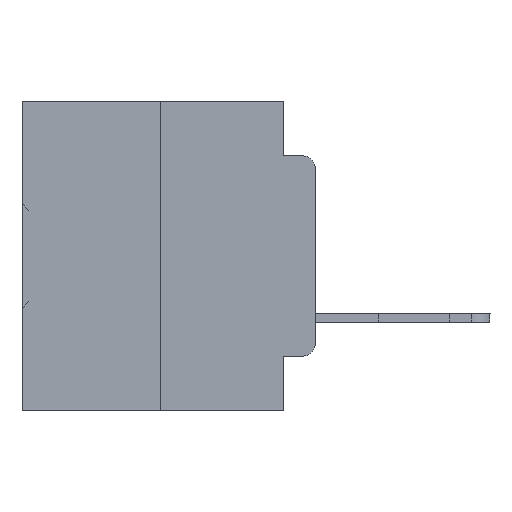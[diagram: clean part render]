
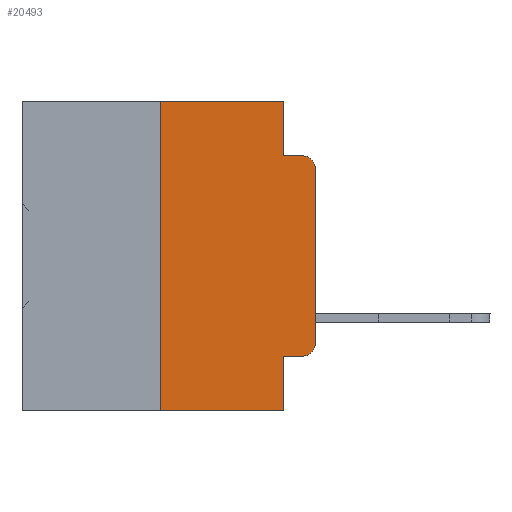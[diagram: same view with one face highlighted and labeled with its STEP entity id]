
A CAD part, left-side view. The second image highlights one B-rep face of the part: STEP entity #20493.
In plain terms, the highlighted planar face has unit normal (-1, 0, 0).
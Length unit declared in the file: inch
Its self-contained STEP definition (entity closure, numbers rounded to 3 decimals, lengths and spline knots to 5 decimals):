
#1062 = EDGE_CURVE ( 'NONE', #1080, #31317, #7346, .T. ) ;
#1080 = VERTEX_POINT ( 'NONE', #16188 ) ;
#1418 = VERTEX_POINT ( 'NONE', #6391 ) ;
#1622 = ORIENTED_EDGE ( 'NONE', *, *, #22302, .F. ) ;
#2137 = LINE ( 'NONE', #31240, #18151 ) ;
#2166 = CARTESIAN_POINT ( 'NONE',  ( 0., 0.02, -0.1085 ) ) ;
#2655 = ORIENTED_EDGE ( 'NONE', *, *, #32962, .F. ) ;
#3033 = DIRECTION ( 'NONE',  ( 0., -1., 0. ) ) ;
#3649 = ORIENTED_EDGE ( 'NONE', *, *, #21889, .F. ) ;
#4477 = DIRECTION ( 'NONE',  ( 0., 0., 1. ) ) ;
#5012 = DIRECTION ( 'NONE',  ( 0., 0., 1. ) ) ;
#5609 = DIRECTION ( 'NONE',  ( 0., 0., -1. ) ) ;
#5659 = DIRECTION ( 'NONE',  ( -1., 0., 0. ) ) ;
#5760 = EDGE_CURVE ( 'NONE', #37710, #1080, #20827, .T. ) ;
#5964 = DIRECTION ( 'NONE',  ( 0., 0., -1. ) ) ;
#6171 = LINE ( 'NONE', #17882, #10372 ) ;
#6391 = CARTESIAN_POINT ( 'NONE',  ( 0., 0.051, -0.4115 ) ) ;
#7346 = LINE ( 'NONE', #19021, #15452 ) ;
#7853 = VERTEX_POINT ( 'NONE', #30922 ) ;
#8041 = LINE ( 'NONE', #31603, #34232 ) ;
#8723 = DIRECTION ( 'NONE',  ( 0., 0., -1. ) ) ;
#8746 = AXIS2_PLACEMENT_3D ( 'NONE', #30864, #31432, #28547 ) ;
#8863 = LINE ( 'NONE', #20525, #22206 ) ;
#9950 = LINE ( 'NONE', #18746, #20154 ) ;
#10372 = VECTOR ( 'NONE', #23235, 39.37008 ) ;
#10520 = CIRCLE ( 'NONE', #31913, 0.02 ) ;
#10738 = LINE ( 'NONE', #37153, #15723 ) ;
#12020 = ORIENTED_EDGE ( 'NONE', *, *, #20349, .F. ) ;
#12160 = VERTEX_POINT ( 'NONE', #22994 ) ;
#13338 = CARTESIAN_POINT ( 'NONE',  ( 0., 0.051, 0. ) ) ;
#13588 = LINE ( 'NONE', #31182, #22371 ) ;
#15452 = VECTOR ( 'NONE', #4477, 39.37008 ) ;
#15601 = VERTEX_POINT ( 'NONE', #15735 ) ;
#15723 = VECTOR ( 'NONE', #3033, 39.37008 ) ;
#15735 = CARTESIAN_POINT ( 'NONE',  ( 0., 0.051, -0.0885 ) ) ;
#15758 = ORIENTED_EDGE ( 'NONE', *, *, #5760, .T. ) ;
#16188 = CARTESIAN_POINT ( 'NONE',  ( 0., 0., -0.3915 ) ) ;
#16746 = VERTEX_POINT ( 'NONE', #35636 ) ;
#16987 = EDGE_CURVE ( 'NONE', #30671, #15601, #8041, .T. ) ;
#17213 = EDGE_CURVE ( 'NONE', #16746, #18371, #9950, .T. ) ;
#17882 = CARTESIAN_POINT ( 'NONE',  ( 0., 0.051, -0.4115 ) ) ;
#18151 = VECTOR ( 'NONE', #5012, 39.37008 ) ;
#18371 = VERTEX_POINT ( 'NONE', #33491 ) ;
#18746 = CARTESIAN_POINT ( 'NONE',  ( 0., 0.473, -0.5 ) ) ;
#19021 = CARTESIAN_POINT ( 'NONE',  ( 0., 0., 0. ) ) ;
#20154 = VECTOR ( 'NONE', #27558, 39.37008 ) ;
#20349 = EDGE_CURVE ( 'NONE', #1418, #18371, #8863, .T. ) ;
#20493 = ADVANCED_FACE ( 'NONE', ( #24374 ), #22432, .F. ) ;
#20525 = CARTESIAN_POINT ( 'NONE',  ( 0., 0.051, 0. ) ) ;
#20827 = CIRCLE ( 'NONE', #30630, 0.02 ) ;
#21889 = EDGE_CURVE ( 'NONE', #16746, #12160, #2137, .T. ) ;
#22206 = VECTOR ( 'NONE', #5964, 39.37008 ) ;
#22302 = EDGE_CURVE ( 'NONE', #12160, #30671, #10738, .T. ) ;
#22344 = ORIENTED_EDGE ( 'NONE', *, *, #16987, .F. ) ;
#22371 = VECTOR ( 'NONE', #27963, 39.37008 ) ;
#22432 = PLANE ( 'NONE',  #8746 ) ;
#22994 = CARTESIAN_POINT ( 'NONE',  ( 0., 0.25, 0. ) ) ;
#23172 = ORIENTED_EDGE ( 'NONE', *, *, #1062, .T. ) ;
#23235 = DIRECTION ( 'NONE',  ( 0., -1., 0. ) ) ;
#24186 = CARTESIAN_POINT ( 'NONE',  ( 0., 0., -0.1085 ) ) ;
#24374 = FACE_OUTER_BOUND ( 'NONE', #28136, .T. ) ;
#25490 = ORIENTED_EDGE ( 'NONE', *, *, #17213, .T. ) ;
#27384 = ORIENTED_EDGE ( 'NONE', *, *, #34170, .T. ) ;
#27558 = DIRECTION ( 'NONE',  ( 0., -1., 0. ) ) ;
#27963 = DIRECTION ( 'NONE',  ( 0., -1., 0. ) ) ;
#28136 = EDGE_LOOP ( 'NONE', ( #23172, #36895, #2655, #22344, #1622, #3649, #25490, #12020, #27384, #15758 ) ) ;
#28547 = DIRECTION ( 'NONE',  ( 0., 0., -1. ) ) ;
#30010 = EDGE_CURVE ( 'NONE', #31317, #7853, #10520, .T. ) ;
#30630 = AXIS2_PLACEMENT_3D ( 'NONE', #37284, #5659, #8723 ) ;
#30671 = VERTEX_POINT ( 'NONE', #13338 ) ;
#30864 = CARTESIAN_POINT ( 'NONE',  ( 0., 0.473, 0. ) ) ;
#30922 = CARTESIAN_POINT ( 'NONE',  ( 0., 0.02, -0.0885 ) ) ;
#31182 = CARTESIAN_POINT ( 'NONE',  ( 0., 0.051, -0.0885 ) ) ;
#31240 = CARTESIAN_POINT ( 'NONE',  ( 0., 0.25, 0. ) ) ;
#31317 = VERTEX_POINT ( 'NONE', #24186 ) ;
#31353 = CARTESIAN_POINT ( 'NONE',  ( 0., 0.02, -0.4115 ) ) ;
#31432 = DIRECTION ( 'NONE',  ( 1., 0., 0. ) ) ;
#31603 = CARTESIAN_POINT ( 'NONE',  ( 0., 0.051, 0. ) ) ;
#31913 = AXIS2_PLACEMENT_3D ( 'NONE', #2166, #34153, #5609 ) ;
#32962 = EDGE_CURVE ( 'NONE', #15601, #7853, #13588, .T. ) ;
#33491 = CARTESIAN_POINT ( 'NONE',  ( 0., 0.051, -0.5 ) ) ;
#34153 = DIRECTION ( 'NONE',  ( -1., 0., 0. ) ) ;
#34170 = EDGE_CURVE ( 'NONE', #1418, #37710, #6171, .T. ) ;
#34232 = VECTOR ( 'NONE', #34841, 39.37008 ) ;
#34841 = DIRECTION ( 'NONE',  ( 0., 0., -1. ) ) ;
#35636 = CARTESIAN_POINT ( 'NONE',  ( 0., 0.25, -0.5 ) ) ;
#36895 = ORIENTED_EDGE ( 'NONE', *, *, #30010, .T. ) ;
#37153 = CARTESIAN_POINT ( 'NONE',  ( 0., 0.473, 0. ) ) ;
#37284 = CARTESIAN_POINT ( 'NONE',  ( 0., 0.02, -0.3915 ) ) ;
#37710 = VERTEX_POINT ( 'NONE', #31353 ) ;
